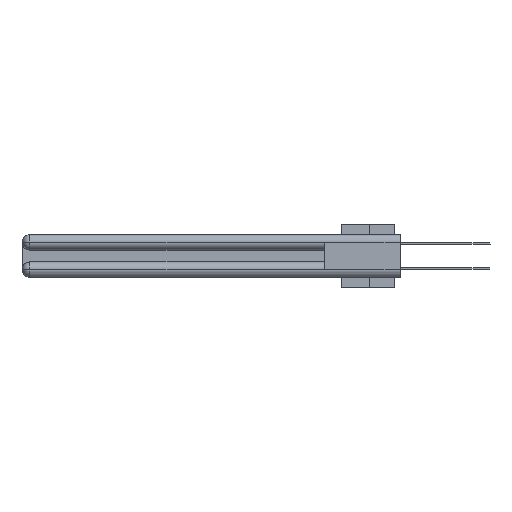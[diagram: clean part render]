
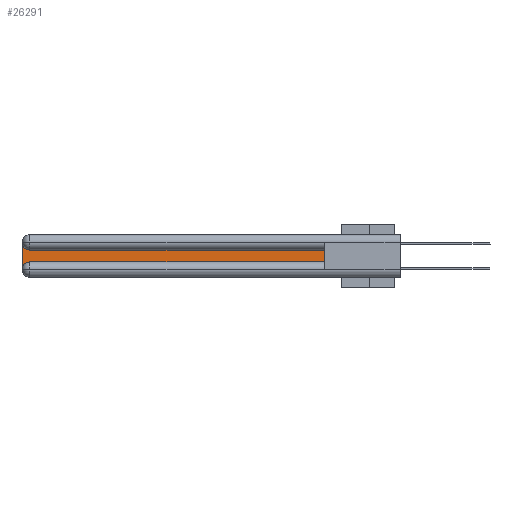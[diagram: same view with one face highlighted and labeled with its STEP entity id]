
A CAD part, left-side view. The second image highlights one B-rep face of the part: STEP entity #26291.
In plain terms, the highlighted planar face has unit normal (-1, 0, 0).
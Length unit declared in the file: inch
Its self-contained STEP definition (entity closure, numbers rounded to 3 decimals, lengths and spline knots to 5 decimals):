
#663 = DIRECTION ( 'NONE',  ( 1., 0., 0. ) ) ;
#2114 = CARTESIAN_POINT ( 'NONE',  ( 0.075, 3., -0.0625 ) ) ;
#2169 = VERTEX_POINT ( 'NONE', #13020 ) ;
#2492 = DIRECTION ( 'NONE',  ( 0., -1., 0. ) ) ;
#2542 = DIRECTION ( 'NONE',  ( 0., 0., -1. ) ) ;
#2882 = DIRECTION ( 'NONE',  ( 1., 0., 0. ) ) ;
#4143 = LINE ( 'NONE', #9540, #8323 ) ;
#4462 = CARTESIAN_POINT ( 'NONE',  ( 0.075, 3., -0.2775 ) ) ;
#5842 = ORIENTED_EDGE ( 'NONE', *, *, #17492, .T. ) ;
#6221 = LINE ( 'NONE', #18364, #33802 ) ;
#7780 = DIRECTION ( 'NONE',  ( 0., 0., 1. ) ) ;
#8323 = VECTOR ( 'NONE', #31027, 39.37008 ) ;
#8608 = PLANE ( 'NONE',  #28541 ) ;
#8816 = VERTEX_POINT ( 'NONE', #4462 ) ;
#9540 = CARTESIAN_POINT ( 'NONE',  ( 0.075, 0.6, -0.1225 ) ) ;
#9840 = CARTESIAN_POINT ( 'NONE',  ( 0.075, 2.94, -0.2175 ) ) ;
#9886 = CIRCLE ( 'NONE', #28858, 0.06 ) ;
#10809 = LINE ( 'NONE', #24102, #30455 ) ;
#10958 = DIRECTION ( 'NONE',  ( 0., 0., -1. ) ) ;
#11337 = DIRECTION ( 'NONE',  ( 0., 0., -1. ) ) ;
#13020 = CARTESIAN_POINT ( 'NONE',  ( 0.075, 2.94, -0.1225 ) ) ;
#13114 = EDGE_CURVE ( 'NONE', #8816, #27685, #9886, .T. ) ;
#14133 = DIRECTION ( 'NONE',  ( 1., 0., 0. ) ) ;
#14286 = LINE ( 'NONE', #26196, #27720 ) ;
#14790 = ORIENTED_EDGE ( 'NONE', *, *, #24678, .T. ) ;
#16429 = CARTESIAN_POINT ( 'NONE',  ( 0.075, 3., -0.1225 ) ) ;
#17024 = AXIS2_PLACEMENT_3D ( 'NONE', #24553, #14133, #11337 ) ;
#17485 = VERTEX_POINT ( 'NONE', #20245 ) ;
#17492 = EDGE_CURVE ( 'NONE', #17860, #2169, #4143, .T. ) ;
#17742 = EDGE_CURVE ( 'NONE', #27685, #17485, #6221, .T. ) ;
#17785 = EDGE_CURVE ( 'NONE', #17485, #17860, #10809, .T. ) ;
#17787 = ORIENTED_EDGE ( 'NONE', *, *, #13114, .T. ) ;
#17860 = VERTEX_POINT ( 'NONE', #30045 ) ;
#18364 = CARTESIAN_POINT ( 'NONE',  ( 0.075, 0.6, -0.2175 ) ) ;
#19118 = CIRCLE ( 'NONE', #17024, 0.06 ) ;
#19335 = ORIENTED_EDGE ( 'NONE', *, *, #17742, .T. ) ;
#20245 = CARTESIAN_POINT ( 'NONE',  ( 0.075, 0.6, -0.2175 ) ) ;
#20251 = FACE_OUTER_BOUND ( 'NONE', #29733, .T. ) ;
#21687 = CARTESIAN_POINT ( 'NONE',  ( 0.075, 2.94, -0.2775 ) ) ;
#23045 = ORIENTED_EDGE ( 'NONE', *, *, #17785, .T. ) ;
#24102 = CARTESIAN_POINT ( 'NONE',  ( 0.075, 0.6, -0.2175 ) ) ;
#24553 = CARTESIAN_POINT ( 'NONE',  ( 0.075, 2.94, -0.0625 ) ) ;
#24678 = EDGE_CURVE ( 'NONE', #2169, #32159, #19118, .T. ) ;
#26196 = CARTESIAN_POINT ( 'NONE',  ( 0.075, 3., -0.2175 ) ) ;
#26291 = ADVANCED_FACE ( 'NONE', ( #20251 ), #8608, .F. ) ;
#26831 = ORIENTED_EDGE ( 'NONE', *, *, #27821, .T. ) ;
#27685 = VERTEX_POINT ( 'NONE', #9840 ) ;
#27720 = VECTOR ( 'NONE', #2542, 39.37008 ) ;
#27821 = EDGE_CURVE ( 'NONE', #32159, #8816, #14286, .T. ) ;
#28541 = AXIS2_PLACEMENT_3D ( 'NONE', #16429, #663, #29981 ) ;
#28858 = AXIS2_PLACEMENT_3D ( 'NONE', #21687, #2882, #10958 ) ;
#29733 = EDGE_LOOP ( 'NONE', ( #5842, #14790, #26831, #17787, #19335, #23045 ) ) ;
#29981 = DIRECTION ( 'NONE',  ( 0., 0., -1. ) ) ;
#30045 = CARTESIAN_POINT ( 'NONE',  ( 0.075, 0.6, -0.1225 ) ) ;
#30455 = VECTOR ( 'NONE', #7780, 39.37008 ) ;
#31027 = DIRECTION ( 'NONE',  ( 0., 1., 0. ) ) ;
#32159 = VERTEX_POINT ( 'NONE', #2114 ) ;
#33802 = VECTOR ( 'NONE', #2492, 39.37008 ) ;
